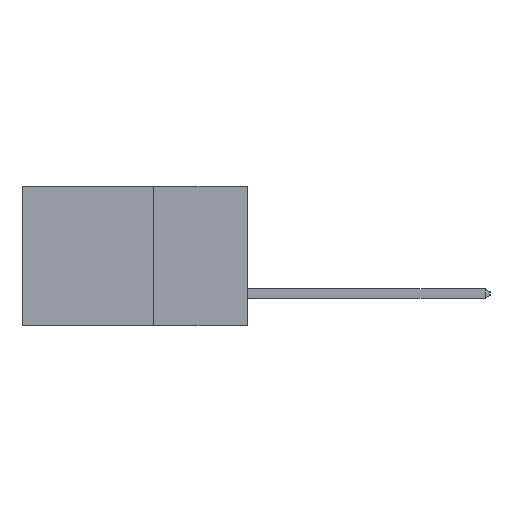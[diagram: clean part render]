
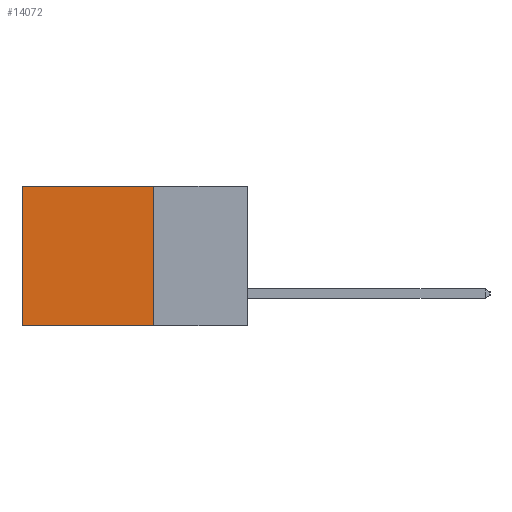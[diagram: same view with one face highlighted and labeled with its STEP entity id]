
A CAD part, left-side view. The second image highlights one B-rep face of the part: STEP entity #14072.
In plain terms, the highlighted planar face has unit normal (-1, 0, 0).
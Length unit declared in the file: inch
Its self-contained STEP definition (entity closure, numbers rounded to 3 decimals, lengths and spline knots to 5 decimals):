
#784 = DIRECTION ( 'NONE',  ( 0., 0., -1. ) ) ;
#969 = DIRECTION ( 'NONE',  ( 1., 0., 0. ) ) ;
#976 = VECTOR ( 'NONE', #13543, 39.37008 ) ;
#1042 = CARTESIAN_POINT ( 'NONE',  ( 0.2615, 0.6, -0.37 ) ) ;
#1306 = LINE ( 'NONE', #1042, #12954 ) ;
#1437 = DIRECTION ( 'NONE',  ( 0., 0., -1. ) ) ;
#2218 = VECTOR ( 'NONE', #11059, 39.37008 ) ;
#3113 = CARTESIAN_POINT ( 'NONE',  ( 0.2615, 0.25, -0.37 ) ) ;
#3452 = LINE ( 'NONE', #12466, #976 ) ;
#4682 = FACE_OUTER_BOUND ( 'NONE', #8777, .T. ) ;
#4701 = VERTEX_POINT ( 'NONE', #8641 ) ;
#5135 = EDGE_CURVE ( 'NONE', #4701, #9192, #1306, .T. ) ;
#6055 = CARTESIAN_POINT ( 'NONE',  ( 0.2615, 0.25, -0.37 ) ) ;
#6504 = ORIENTED_EDGE ( 'NONE', *, *, #10695, .F. ) ;
#6600 = VECTOR ( 'NONE', #1437, 39.37008 ) ;
#7540 = VERTEX_POINT ( 'NONE', #9722 ) ;
#8641 = CARTESIAN_POINT ( 'NONE',  ( 0.2615, 0.6, 0. ) ) ;
#8777 = EDGE_LOOP ( 'NONE', ( #10712, #6504, #12652, #14032 ) ) ;
#9066 = DIRECTION ( 'NONE',  ( 0., 0., -1. ) ) ;
#9192 = VERTEX_POINT ( 'NONE', #13678 ) ;
#9579 = LINE ( 'NONE', #6055, #6600 ) ;
#9722 = CARTESIAN_POINT ( 'NONE',  ( 0.2615, 0.25, 0. ) ) ;
#9975 = VERTEX_POINT ( 'NONE', #3113 ) ;
#10377 = EDGE_CURVE ( 'NONE', #7540, #9975, #9579, .T. ) ;
#10695 = EDGE_CURVE ( 'NONE', #9975, #9192, #11275, .T. ) ;
#10712 = ORIENTED_EDGE ( 'NONE', *, *, #5135, .T. ) ;
#11059 = DIRECTION ( 'NONE',  ( 0., 1., 0. ) ) ;
#11275 = LINE ( 'NONE', #13183, #2218 ) ;
#12248 = PLANE ( 'NONE',  #12260 ) ;
#12260 = AXIS2_PLACEMENT_3D ( 'NONE', #13299, #969, #9066 ) ;
#12466 = CARTESIAN_POINT ( 'NONE',  ( 0.2615, 0.25, 0. ) ) ;
#12652 = ORIENTED_EDGE ( 'NONE', *, *, #10377, .F. ) ;
#12954 = VECTOR ( 'NONE', #784, 39.37008 ) ;
#13183 = CARTESIAN_POINT ( 'NONE',  ( 0.2615, 0.25, -0.37 ) ) ;
#13299 = CARTESIAN_POINT ( 'NONE',  ( 0.2615, 0.25, -0.37 ) ) ;
#13530 = EDGE_CURVE ( 'NONE', #7540, #4701, #3452, .T. ) ;
#13543 = DIRECTION ( 'NONE',  ( 0., 1., 0. ) ) ;
#13678 = CARTESIAN_POINT ( 'NONE',  ( 0.2615, 0.6, -0.37 ) ) ;
#14032 = ORIENTED_EDGE ( 'NONE', *, *, #13530, .T. ) ;
#14072 = ADVANCED_FACE ( 'NONE', ( #4682 ), #12248, .F. ) ;
